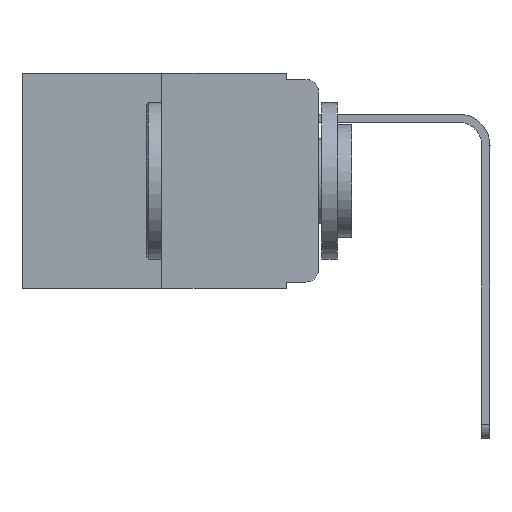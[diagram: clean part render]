
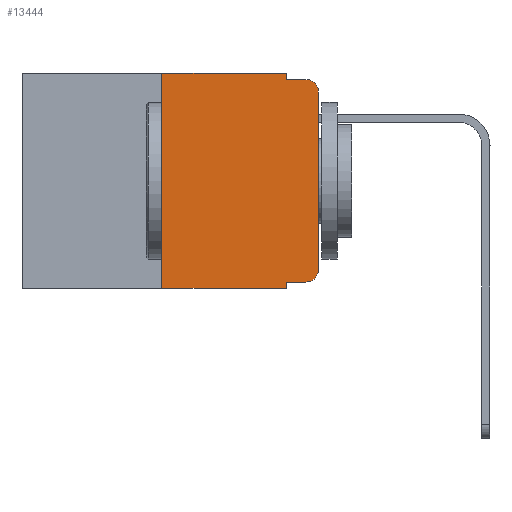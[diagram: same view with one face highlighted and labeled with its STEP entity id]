
A CAD part, left-side view. The second image highlights one B-rep face of the part: STEP entity #13444.
In plain terms, the highlighted planar face has unit normal (-1, 0, 0).
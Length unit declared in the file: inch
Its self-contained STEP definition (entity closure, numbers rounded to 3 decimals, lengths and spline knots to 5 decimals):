
#277 = CARTESIAN_POINT ( 'NONE',  ( 0., 0.02, -0.333 ) ) ;
#709 = VERTEX_POINT ( 'NONE', #13683 ) ;
#1833 = CARTESIAN_POINT ( 'NONE',  ( 0., 0.02, -0.313 ) ) ;
#1918 = DIRECTION ( 'NONE',  ( 0., -1., 0. ) ) ;
#2239 = CARTESIAN_POINT ( 'NONE',  ( 0., 0.051, 0. ) ) ;
#2497 = VECTOR ( 'NONE', #5253, 39.37008 ) ;
#3024 = LINE ( 'NONE', #2239, #24215 ) ;
#3124 = LINE ( 'NONE', #17308, #2497 ) ;
#3423 = CARTESIAN_POINT ( 'NONE',  ( 0., 0.25, 0. ) ) ;
#3492 = CARTESIAN_POINT ( 'NONE',  ( 0., 0.051, -0.01 ) ) ;
#3752 = CIRCLE ( 'NONE', #18557, 0.02 ) ;
#3961 = ORIENTED_EDGE ( 'NONE', *, *, #9004, .F. ) ;
#3963 = DIRECTION ( 'NONE',  ( 0., 0., -1. ) ) ;
#3977 = ORIENTED_EDGE ( 'NONE', *, *, #18080, .T. ) ;
#3980 = VERTEX_POINT ( 'NONE', #12517 ) ;
#4026 = ORIENTED_EDGE ( 'NONE', *, *, #16047, .T. ) ;
#4508 = ORIENTED_EDGE ( 'NONE', *, *, #14973, .F. ) ;
#4945 = ORIENTED_EDGE ( 'NONE', *, *, #10574, .T. ) ;
#5253 = DIRECTION ( 'NONE',  ( 0., 0., 1. ) ) ;
#5425 = LINE ( 'NONE', #3492, #20892 ) ;
#5505 = DIRECTION ( 'NONE',  ( 0., -1., 0. ) ) ;
#5915 = CARTESIAN_POINT ( 'NONE',  ( 0., 0.051, 0. ) ) ;
#6094 = DIRECTION ( 'NONE',  ( 0., -1., 0. ) ) ;
#6168 = CARTESIAN_POINT ( 'NONE',  ( 0., 0.051, -0.01 ) ) ;
#7093 = VECTOR ( 'NONE', #24258, 39.37008 ) ;
#7727 = LINE ( 'NONE', #5915, #7093 ) ;
#7812 = EDGE_CURVE ( 'NONE', #11170, #12146, #3024, .T. ) ;
#7956 = VECTOR ( 'NONE', #6094, 39.37008 ) ;
#7998 = CARTESIAN_POINT ( 'NONE',  ( 0., 0., 0. ) ) ;
#8017 = DIRECTION ( 'NONE',  ( 0., 0., -1. ) ) ;
#8441 = DIRECTION ( 'NONE',  ( 0., 0., -1. ) ) ;
#9004 = EDGE_CURVE ( 'NONE', #19309, #21164, #7727, .T. ) ;
#9193 = ORIENTED_EDGE ( 'NONE', *, *, #10193, .T. ) ;
#9599 = ORIENTED_EDGE ( 'NONE', *, *, #22623, .F. ) ;
#10193 = EDGE_CURVE ( 'NONE', #25508, #3980, #20276, .T. ) ;
#10574 = EDGE_CURVE ( 'NONE', #19309, #25508, #22445, .T. ) ;
#10627 = CARTESIAN_POINT ( 'NONE',  ( 0., 0.051, -0.343 ) ) ;
#10810 = LINE ( 'NONE', #19918, #7956 ) ;
#11170 = VERTEX_POINT ( 'NONE', #13474 ) ;
#11563 = DIRECTION ( 'NONE',  ( 0., -1., 0. ) ) ;
#12146 = VERTEX_POINT ( 'NONE', #6168 ) ;
#12347 = VERTEX_POINT ( 'NONE', #14799 ) ;
#12517 = CARTESIAN_POINT ( 'NONE',  ( 0., 0., -0.313 ) ) ;
#12564 = CARTESIAN_POINT ( 'NONE',  ( 0., 0.02, -0.03 ) ) ;
#13444 = ADVANCED_FACE ( 'NONE', ( #17471 ), #14307, .F. ) ;
#13474 = CARTESIAN_POINT ( 'NONE',  ( 0., 0.051, 0. ) ) ;
#13683 = CARTESIAN_POINT ( 'NONE',  ( 0., 0., -0.03 ) ) ;
#14307 = PLANE ( 'NONE',  #18862 ) ;
#14398 = CARTESIAN_POINT ( 'NONE',  ( 0., 0.473, 0. ) ) ;
#14505 = DIRECTION ( 'NONE',  ( 0., 0., -1. ) ) ;
#14799 = CARTESIAN_POINT ( 'NONE',  ( 0., 0.25, -0.343 ) ) ;
#14973 = EDGE_CURVE ( 'NONE', #12146, #20062, #5425, .T. ) ;
#15171 = VECTOR ( 'NONE', #23871, 39.37008 ) ;
#15181 = CARTESIAN_POINT ( 'NONE',  ( 0., 0.051, -0.333 ) ) ;
#15956 = DIRECTION ( 'NONE',  ( -1., 0., 0. ) ) ;
#16047 = EDGE_CURVE ( 'NONE', #709, #20062, #3752, .T. ) ;
#16202 = CARTESIAN_POINT ( 'NONE',  ( 0., 0.02, -0.01 ) ) ;
#16847 = ORIENTED_EDGE ( 'NONE', *, *, #18602, .F. ) ;
#17308 = CARTESIAN_POINT ( 'NONE',  ( 0., 0.25, 0. ) ) ;
#17466 = VECTOR ( 'NONE', #5505, 39.37008 ) ;
#17471 = FACE_OUTER_BOUND ( 'NONE', #25910, .T. ) ;
#17576 = CARTESIAN_POINT ( 'NONE',  ( 0., 0.473, 0. ) ) ;
#17804 = CARTESIAN_POINT ( 'NONE',  ( 0., 0.051, -0.333 ) ) ;
#18080 = EDGE_CURVE ( 'NONE', #3980, #709, #23055, .T. ) ;
#18093 = DIRECTION ( 'NONE',  ( 1., 0., 0. ) ) ;
#18361 = VECTOR ( 'NONE', #1918, 39.37008 ) ;
#18557 = AXIS2_PLACEMENT_3D ( 'NONE', #12564, #24380, #14505 ) ;
#18602 = EDGE_CURVE ( 'NONE', #12347, #21349, #3124, .T. ) ;
#18862 = AXIS2_PLACEMENT_3D ( 'NONE', #14398, #18093, #3963 ) ;
#19309 = VERTEX_POINT ( 'NONE', #15181 ) ;
#19918 = CARTESIAN_POINT ( 'NONE',  ( 0., 0.473, -0.343 ) ) ;
#20062 = VERTEX_POINT ( 'NONE', #16202 ) ;
#20276 = CIRCLE ( 'NONE', #24308, 0.02 ) ;
#20892 = VECTOR ( 'NONE', #11563, 39.37008 ) ;
#21164 = VERTEX_POINT ( 'NONE', #10627 ) ;
#21257 = LINE ( 'NONE', #17576, #17466 ) ;
#21349 = VERTEX_POINT ( 'NONE', #3423 ) ;
#22291 = ORIENTED_EDGE ( 'NONE', *, *, #23405, .T. ) ;
#22445 = LINE ( 'NONE', #17804, #18361 ) ;
#22623 = EDGE_CURVE ( 'NONE', #21349, #11170, #21257, .T. ) ;
#23055 = LINE ( 'NONE', #7998, #15171 ) ;
#23405 = EDGE_CURVE ( 'NONE', #12347, #21164, #10810, .T. ) ;
#23871 = DIRECTION ( 'NONE',  ( 0., 0., 1. ) ) ;
#24215 = VECTOR ( 'NONE', #8441, 39.37008 ) ;
#24258 = DIRECTION ( 'NONE',  ( 0., 0., -1. ) ) ;
#24308 = AXIS2_PLACEMENT_3D ( 'NONE', #1833, #15956, #8017 ) ;
#24380 = DIRECTION ( 'NONE',  ( -1., 0., 0. ) ) ;
#25508 = VERTEX_POINT ( 'NONE', #277 ) ;
#25660 = ORIENTED_EDGE ( 'NONE', *, *, #7812, .F. ) ;
#25910 = EDGE_LOOP ( 'NONE', ( #3977, #4026, #4508, #25660, #9599, #16847, #22291, #3961, #4945, #9193 ) ) ;
